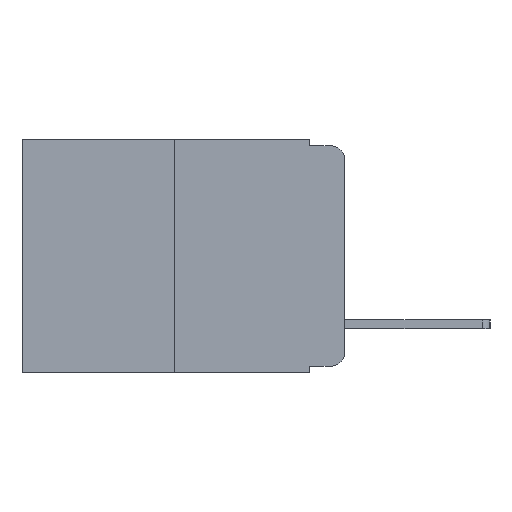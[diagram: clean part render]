
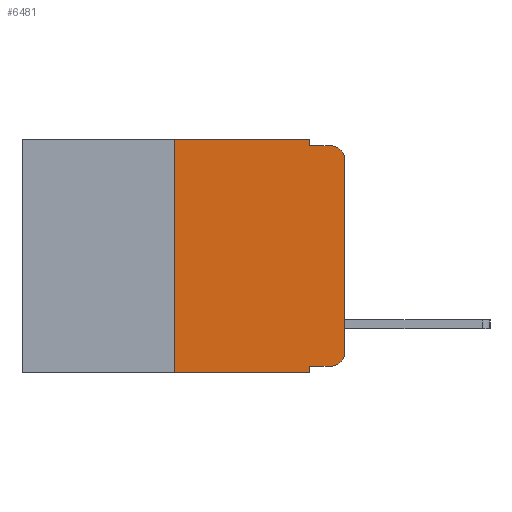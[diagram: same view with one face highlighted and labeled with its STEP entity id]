
A CAD part, left-side view. The second image highlights one B-rep face of the part: STEP entity #6481.
In plain terms, the highlighted planar face has unit normal (-1, 0, 0).
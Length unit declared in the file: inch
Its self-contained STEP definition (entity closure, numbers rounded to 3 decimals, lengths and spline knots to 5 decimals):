
#65 = ORIENTED_EDGE ( 'NONE', *, *, #17061, .F. ) ;
#843 = EDGE_CURVE ( 'NONE', #17377, #5470, #15962, .T. ) ;
#850 = ORIENTED_EDGE ( 'NONE', *, *, #19107, .T. ) ;
#980 = DIRECTION ( 'NONE',  ( -1., 0., 0. ) ) ;
#1017 = CARTESIAN_POINT ( 'NONE',  ( 0., 0.051, 0. ) ) ;
#1056 = ORIENTED_EDGE ( 'NONE', *, *, #5787, .T. ) ;
#1087 = VECTOR ( 'NONE', #7430, 39.37008 ) ;
#1147 = CARTESIAN_POINT ( 'NONE',  ( 0., 0., -0.313 ) ) ;
#1213 = LINE ( 'NONE', #3335, #17434 ) ;
#1961 = DIRECTION ( 'NONE',  ( 0., -1., 0. ) ) ;
#2376 = CARTESIAN_POINT ( 'NONE',  ( 0., 0.473, 0. ) ) ;
#2430 = CARTESIAN_POINT ( 'NONE',  ( 0., 0.051, -0.01 ) ) ;
#2471 = CARTESIAN_POINT ( 'NONE',  ( 0., 0.25, -0.343 ) ) ;
#2662 = CARTESIAN_POINT ( 'NONE',  ( 0., 0.051, -0.343 ) ) ;
#3246 = ORIENTED_EDGE ( 'NONE', *, *, #10891, .T. ) ;
#3335 = CARTESIAN_POINT ( 'NONE',  ( 0., 0.473, -0.343 ) ) ;
#3647 = DIRECTION ( 'NONE',  ( 0., 0., 1. ) ) ;
#4514 = CARTESIAN_POINT ( 'NONE',  ( 0., 0.02, -0.313 ) ) ;
#4540 = LINE ( 'NONE', #12996, #8271 ) ;
#4829 = CARTESIAN_POINT ( 'NONE',  ( 0., 0.051, 0. ) ) ;
#4867 = LINE ( 'NONE', #10606, #1087 ) ;
#5137 = CARTESIAN_POINT ( 'NONE',  ( 0., 0., 0. ) ) ;
#5194 = LINE ( 'NONE', #4829, #8924 ) ;
#5399 = VECTOR ( 'NONE', #6432, 39.37008 ) ;
#5470 = VERTEX_POINT ( 'NONE', #13138 ) ;
#5787 = EDGE_CURVE ( 'NONE', #17796, #15469, #1213, .T. ) ;
#6417 = ORIENTED_EDGE ( 'NONE', *, *, #13951, .F. ) ;
#6432 = DIRECTION ( 'NONE',  ( 0., 0., 1. ) ) ;
#6434 = DIRECTION ( 'NONE',  ( 0., 0., -1. ) ) ;
#6481 = ADVANCED_FACE ( 'NONE', ( #20159 ), #14699, .F. ) ;
#6892 = VERTEX_POINT ( 'NONE', #13556 ) ;
#7110 = LINE ( 'NONE', #1017, #18969 ) ;
#7430 = DIRECTION ( 'NONE',  ( 0., -1., 0. ) ) ;
#7465 = CARTESIAN_POINT ( 'NONE',  ( 0., 0.02, -0.01 ) ) ;
#7553 = AXIS2_PLACEMENT_3D ( 'NONE', #14632, #14500, #8808 ) ;
#8190 = ORIENTED_EDGE ( 'NONE', *, *, #18409, .F. ) ;
#8271 = VECTOR ( 'NONE', #1961, 39.37008 ) ;
#8475 = VERTEX_POINT ( 'NONE', #15995 ) ;
#8808 = DIRECTION ( 'NONE',  ( 0., 0., -1. ) ) ;
#8832 = ORIENTED_EDGE ( 'NONE', *, *, #9821, .T. ) ;
#8894 = CIRCLE ( 'NONE', #17814, 0.02 ) ;
#8924 = VECTOR ( 'NONE', #14205, 39.37008 ) ;
#8999 = DIRECTION ( 'NONE',  ( 0., 0., -1. ) ) ;
#9625 = LINE ( 'NONE', #15731, #5399 ) ;
#9821 = EDGE_CURVE ( 'NONE', #6892, #17377, #8894, .T. ) ;
#10571 = CARTESIAN_POINT ( 'NONE',  ( 0., 0.02, -0.03 ) ) ;
#10606 = CARTESIAN_POINT ( 'NONE',  ( 0., 0.051, -0.333 ) ) ;
#10891 = EDGE_CURVE ( 'NONE', #17216, #6892, #4867, .T. ) ;
#11087 = VECTOR ( 'NONE', #14868, 39.37008 ) ;
#11906 = VECTOR ( 'NONE', #3647, 39.37008 ) ;
#11910 = EDGE_LOOP ( 'NONE', ( #12664, #850, #65, #16143, #8190, #6417, #1056, #14914, #3246, #8832 ) ) ;
#12131 = DIRECTION ( 'NONE',  ( 0., 0., -1. ) ) ;
#12622 = VERTEX_POINT ( 'NONE', #16531 ) ;
#12664 = ORIENTED_EDGE ( 'NONE', *, *, #843, .T. ) ;
#12920 = EDGE_CURVE ( 'NONE', #17216, #15469, #5194, .T. ) ;
#12996 = CARTESIAN_POINT ( 'NONE',  ( 0., 0.051, -0.01 ) ) ;
#13138 = CARTESIAN_POINT ( 'NONE',  ( 0., 0., -0.03 ) ) ;
#13556 = CARTESIAN_POINT ( 'NONE',  ( 0., 0.02, -0.333 ) ) ;
#13698 = AXIS2_PLACEMENT_3D ( 'NONE', #10571, #980, #12131 ) ;
#13951 = EDGE_CURVE ( 'NONE', #17796, #12622, #9625, .T. ) ;
#14205 = DIRECTION ( 'NONE',  ( 0., 0., -1. ) ) ;
#14500 = DIRECTION ( 'NONE',  ( 1., 0., 0. ) ) ;
#14632 = CARTESIAN_POINT ( 'NONE',  ( 0., 0.473, 0. ) ) ;
#14699 = PLANE ( 'NONE',  #7553 ) ;
#14868 = DIRECTION ( 'NONE',  ( 0., -1., 0. ) ) ;
#14869 = CIRCLE ( 'NONE', #13698, 0.02 ) ;
#14914 = ORIENTED_EDGE ( 'NONE', *, *, #12920, .F. ) ;
#14987 = EDGE_CURVE ( 'NONE', #8475, #17723, #7110, .T. ) ;
#15303 = DIRECTION ( 'NONE',  ( 0., -1., 0. ) ) ;
#15466 = DIRECTION ( 'NONE',  ( -1., 0., 0. ) ) ;
#15469 = VERTEX_POINT ( 'NONE', #2662 ) ;
#15731 = CARTESIAN_POINT ( 'NONE',  ( 0., 0.25, 0. ) ) ;
#15962 = LINE ( 'NONE', #5137, #11906 ) ;
#15995 = CARTESIAN_POINT ( 'NONE',  ( 0., 0.051, 0. ) ) ;
#16096 = VERTEX_POINT ( 'NONE', #7465 ) ;
#16143 = ORIENTED_EDGE ( 'NONE', *, *, #14987, .F. ) ;
#16531 = CARTESIAN_POINT ( 'NONE',  ( 0., 0.25, 0. ) ) ;
#17061 = EDGE_CURVE ( 'NONE', #17723, #16096, #4540, .T. ) ;
#17216 = VERTEX_POINT ( 'NONE', #18034 ) ;
#17377 = VERTEX_POINT ( 'NONE', #1147 ) ;
#17434 = VECTOR ( 'NONE', #15303, 39.37008 ) ;
#17723 = VERTEX_POINT ( 'NONE', #2430 ) ;
#17796 = VERTEX_POINT ( 'NONE', #2471 ) ;
#17814 = AXIS2_PLACEMENT_3D ( 'NONE', #4514, #15466, #6434 ) ;
#18034 = CARTESIAN_POINT ( 'NONE',  ( 0., 0.051, -0.333 ) ) ;
#18409 = EDGE_CURVE ( 'NONE', #12622, #8475, #19234, .T. ) ;
#18969 = VECTOR ( 'NONE', #8999, 39.37008 ) ;
#19107 = EDGE_CURVE ( 'NONE', #5470, #16096, #14869, .T. ) ;
#19234 = LINE ( 'NONE', #2376, #11087 ) ;
#20159 = FACE_OUTER_BOUND ( 'NONE', #11910, .T. ) ;
